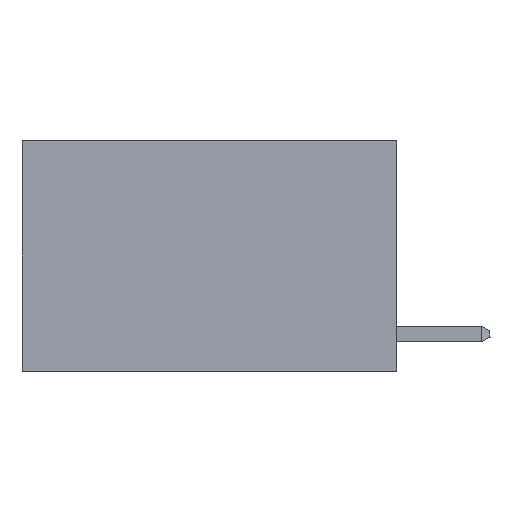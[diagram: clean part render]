
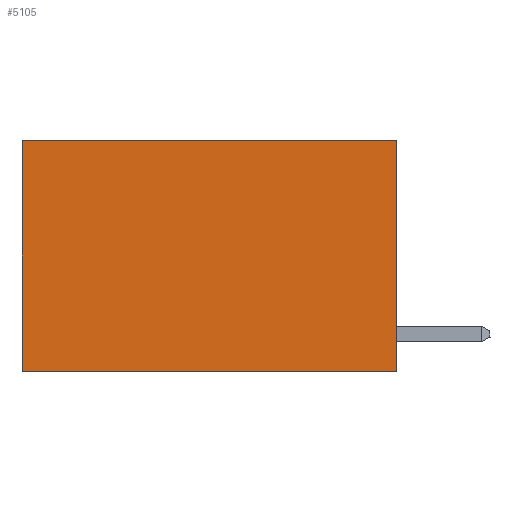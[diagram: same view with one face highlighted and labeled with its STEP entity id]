
A CAD part, left-side view. The second image highlights one B-rep face of the part: STEP entity #5105.
In plain terms, the highlighted planar face has unit normal (-1, 0, 0).
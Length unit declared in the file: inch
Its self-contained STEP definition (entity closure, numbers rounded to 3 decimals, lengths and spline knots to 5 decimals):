
#208 = VERTEX_POINT ( 'NONE', #3153 ) ;
#411 = DIRECTION ( 'NONE',  ( 1., 0., 0. ) ) ;
#576 = LINE ( 'NONE', #7940, #6148 ) ;
#707 = VECTOR ( 'NONE', #6605, 39.37008 ) ;
#776 = ORIENTED_EDGE ( 'NONE', *, *, #5913, .F. ) ;
#2104 = DIRECTION ( 'NONE',  ( 0., 0., -1. ) ) ;
#2243 = CARTESIAN_POINT ( 'NONE',  ( 0.2625, 0., -0.37 ) ) ;
#2496 = CARTESIAN_POINT ( 'NONE',  ( 0.2625, 0., 0. ) ) ;
#3037 = DIRECTION ( 'NONE',  ( 0., 0., -1. ) ) ;
#3153 = CARTESIAN_POINT ( 'NONE',  ( 0.2625, 0., 0. ) ) ;
#3398 = VECTOR ( 'NONE', #4955, 39.37008 ) ;
#3803 = EDGE_CURVE ( 'NONE', #5560, #7760, #6145, .T. ) ;
#4166 = EDGE_LOOP ( 'NONE', ( #6255, #8815, #776, #4949 ) ) ;
#4267 = CARTESIAN_POINT ( 'NONE',  ( 0.2625, 0., 0. ) ) ;
#4528 = VERTEX_POINT ( 'NONE', #2243 ) ;
#4942 = VECTOR ( 'NONE', #2104, 39.37008 ) ;
#4949 = ORIENTED_EDGE ( 'NONE', *, *, #7717, .T. ) ;
#4955 = DIRECTION ( 'NONE',  ( 0., 0., -1. ) ) ;
#5004 = CARTESIAN_POINT ( 'NONE',  ( 0.2625, 0.6, 0. ) ) ;
#5015 = CARTESIAN_POINT ( 'NONE',  ( 0.2625, 0.6, -0.37 ) ) ;
#5105 = ADVANCED_FACE ( 'NONE', ( #6512 ), #7781, .F. ) ;
#5560 = VERTEX_POINT ( 'NONE', #5004 ) ;
#5798 = CARTESIAN_POINT ( 'NONE',  ( 0.2625, 0., 0. ) ) ;
#5913 = EDGE_CURVE ( 'NONE', #208, #4528, #7022, .T. ) ;
#6115 = CARTESIAN_POINT ( 'NONE',  ( 0.2625, 0.6, 0. ) ) ;
#6145 = LINE ( 'NONE', #6115, #4942 ) ;
#6148 = VECTOR ( 'NONE', #6687, 39.37008 ) ;
#6255 = ORIENTED_EDGE ( 'NONE', *, *, #3803, .T. ) ;
#6512 = FACE_OUTER_BOUND ( 'NONE', #4166, .T. ) ;
#6605 = DIRECTION ( 'NONE',  ( 0., 1., 0. ) ) ;
#6687 = DIRECTION ( 'NONE',  ( 0., 1., 0. ) ) ;
#7022 = LINE ( 'NONE', #4267, #3398 ) ;
#7092 = AXIS2_PLACEMENT_3D ( 'NONE', #5798, #411, #3037 ) ;
#7717 = EDGE_CURVE ( 'NONE', #208, #5560, #8625, .T. ) ;
#7760 = VERTEX_POINT ( 'NONE', #5015 ) ;
#7781 = PLANE ( 'NONE',  #7092 ) ;
#7940 = CARTESIAN_POINT ( 'NONE',  ( 0.2625, 0., -0.37 ) ) ;
#8625 = LINE ( 'NONE', #2496, #707 ) ;
#8679 = EDGE_CURVE ( 'NONE', #4528, #7760, #576, .T. ) ;
#8815 = ORIENTED_EDGE ( 'NONE', *, *, #8679, .F. ) ;
